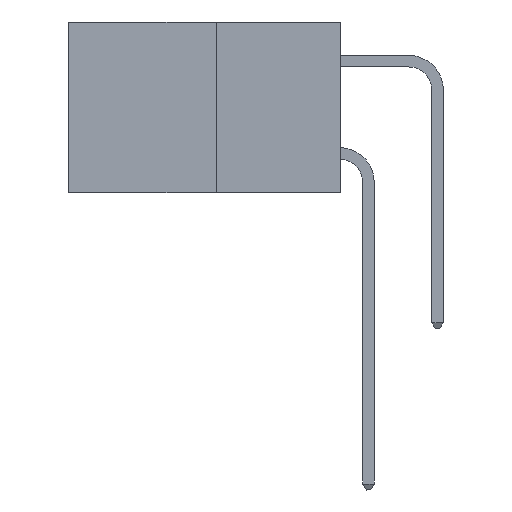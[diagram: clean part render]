
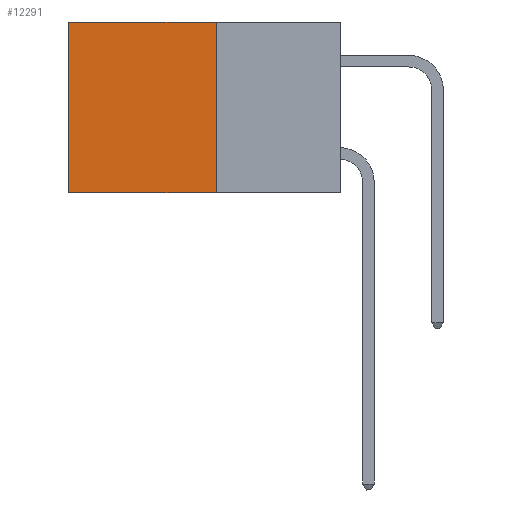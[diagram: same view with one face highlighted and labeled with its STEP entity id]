
A CAD part, left-side view. The second image highlights one B-rep face of the part: STEP entity #12291.
In plain terms, the highlighted planar face has unit normal (-1, 0, 0).
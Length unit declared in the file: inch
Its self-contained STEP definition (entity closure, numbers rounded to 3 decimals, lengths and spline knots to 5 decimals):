
#1200 = CARTESIAN_POINT ( 'NONE',  ( 0.277, 0.27, 0. ) ) ;
#1254 = EDGE_CURVE ( 'NONE', #14066, #33856, #24888, .T. ) ;
#1338 = LINE ( 'NONE', #1200, #22106 ) ;
#1342 = VERTEX_POINT ( 'NONE', #33498 ) ;
#2620 = DIRECTION ( 'NONE',  ( 0., 0., -1. ) ) ;
#3951 = VERTEX_POINT ( 'NONE', #23066 ) ;
#4597 = EDGE_LOOP ( 'NONE', ( #4691, #5334, #15854, #23168 ) ) ;
#4691 = ORIENTED_EDGE ( 'NONE', *, *, #1254, .T. ) ;
#4912 = VECTOR ( 'NONE', #2620, 39.37008 ) ;
#5092 = CARTESIAN_POINT ( 'NONE',  ( 0.277, 0.59, 0. ) ) ;
#5334 = ORIENTED_EDGE ( 'NONE', *, *, #13823, .F. ) ;
#6576 = FACE_OUTER_BOUND ( 'NONE', #4597, .T. ) ;
#6637 = DIRECTION ( 'NONE',  ( 0., 1., 0. ) ) ;
#8682 = CARTESIAN_POINT ( 'NONE',  ( 0.277, 0.59, -0.37 ) ) ;
#10658 = VECTOR ( 'NONE', #25850, 39.37008 ) ;
#12291 = ADVANCED_FACE ( 'NONE', ( #6576 ), #33082, .F. ) ;
#12403 = CARTESIAN_POINT ( 'NONE',  ( 0.277, 0.27, -0.37 ) ) ;
#13823 = EDGE_CURVE ( 'NONE', #1342, #33856, #14883, .T. ) ;
#14066 = VERTEX_POINT ( 'NONE', #5092 ) ;
#14427 = CARTESIAN_POINT ( 'NONE',  ( 0.277, 0.27, -0.37 ) ) ;
#14883 = LINE ( 'NONE', #12403, #21199 ) ;
#15854 = ORIENTED_EDGE ( 'NONE', *, *, #29724, .F. ) ;
#17111 = DIRECTION ( 'NONE',  ( 0., 0., -1. ) ) ;
#19266 = LINE ( 'NONE', #34997, #4912 ) ;
#21199 = VECTOR ( 'NONE', #33916, 39.37008 ) ;
#22106 = VECTOR ( 'NONE', #6637, 39.37008 ) ;
#23066 = CARTESIAN_POINT ( 'NONE',  ( 0.277, 0.27, 0. ) ) ;
#23168 = ORIENTED_EDGE ( 'NONE', *, *, #34763, .T. ) ;
#24888 = LINE ( 'NONE', #29100, #10658 ) ;
#25850 = DIRECTION ( 'NONE',  ( 0., 0., -1. ) ) ;
#29100 = CARTESIAN_POINT ( 'NONE',  ( 0.277, 0.59, -0.37 ) ) ;
#29724 = EDGE_CURVE ( 'NONE', #3951, #1342, #19266, .T. ) ;
#32133 = AXIS2_PLACEMENT_3D ( 'NONE', #14427, #33285, #17111 ) ;
#33082 = PLANE ( 'NONE',  #32133 ) ;
#33285 = DIRECTION ( 'NONE',  ( 1., 0., 0. ) ) ;
#33498 = CARTESIAN_POINT ( 'NONE',  ( 0.277, 0.27, -0.37 ) ) ;
#33856 = VERTEX_POINT ( 'NONE', #8682 ) ;
#33916 = DIRECTION ( 'NONE',  ( 0., 1., 0. ) ) ;
#34763 = EDGE_CURVE ( 'NONE', #3951, #14066, #1338, .T. ) ;
#34997 = CARTESIAN_POINT ( 'NONE',  ( 0.277, 0.27, -0.37 ) ) ;
